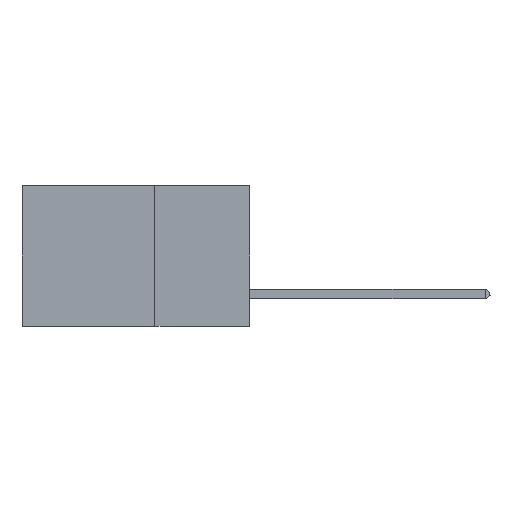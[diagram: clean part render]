
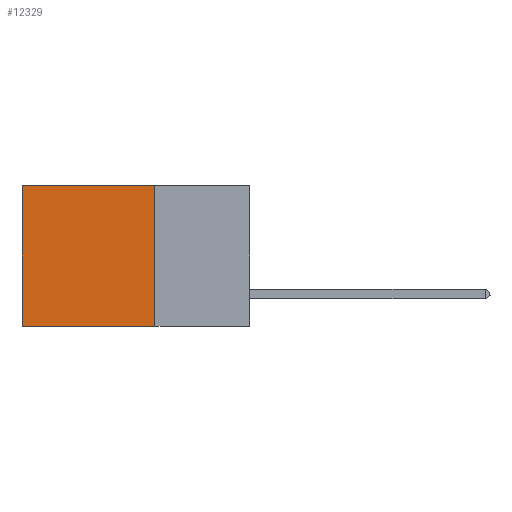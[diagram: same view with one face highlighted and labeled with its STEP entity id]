
A CAD part, left-side view. The second image highlights one B-rep face of the part: STEP entity #12329.
In plain terms, the highlighted planar face has unit normal (-1, 0, 0).
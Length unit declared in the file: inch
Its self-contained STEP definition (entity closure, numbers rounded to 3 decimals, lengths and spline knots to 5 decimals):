
#184 = VECTOR ( 'NONE', #36375, 39.37008 ) ;
#1057 = VERTEX_POINT ( 'NONE', #8124 ) ;
#3148 = AXIS2_PLACEMENT_3D ( 'NONE', #3302, #5001, #36718 ) ;
#3302 = CARTESIAN_POINT ( 'NONE',  ( 0.2875, 0.25, 0. ) ) ;
#3563 = LINE ( 'NONE', #32785, #184 ) ;
#3978 = VERTEX_POINT ( 'NONE', #33314 ) ;
#4868 = DIRECTION ( 'NONE',  ( 0., 0., -1. ) ) ;
#5001 = DIRECTION ( 'NONE',  ( 1., 0., 0. ) ) ;
#5904 = DIRECTION ( 'NONE',  ( 0., 1., 0. ) ) ;
#8124 = CARTESIAN_POINT ( 'NONE',  ( 0.2875, 0.25, -0.37 ) ) ;
#9807 = VERTEX_POINT ( 'NONE', #43853 ) ;
#12329 = ADVANCED_FACE ( 'NONE', ( #24582 ), #19595, .F. ) ;
#13086 = VECTOR ( 'NONE', #5904, 39.37008 ) ;
#13516 = LINE ( 'NONE', #33760, #33788 ) ;
#13643 = VERTEX_POINT ( 'NONE', #44103 ) ;
#16789 = VECTOR ( 'NONE', #41852, 39.37008 ) ;
#19595 = PLANE ( 'NONE',  #3148 ) ;
#22718 = LINE ( 'NONE', #35078, #13086 ) ;
#22846 = EDGE_CURVE ( 'NONE', #3978, #1057, #44266, .T. ) ;
#24582 = FACE_OUTER_BOUND ( 'NONE', #34181, .T. ) ;
#29083 = EDGE_CURVE ( 'NONE', #3978, #9807, #3563, .T. ) ;
#32785 = CARTESIAN_POINT ( 'NONE',  ( 0.2875, 0.25, 0. ) ) ;
#33314 = CARTESIAN_POINT ( 'NONE',  ( 0.2875, 0.25, 0. ) ) ;
#33760 = CARTESIAN_POINT ( 'NONE',  ( 0.2875, 0.6, 0. ) ) ;
#33788 = VECTOR ( 'NONE', #4868, 39.37008 ) ;
#34181 = EDGE_LOOP ( 'NONE', ( #44430, #35342, #35386, #44354 ) ) ;
#35078 = CARTESIAN_POINT ( 'NONE',  ( 0.2875, 0.25, -0.37 ) ) ;
#35342 = ORIENTED_EDGE ( 'NONE', *, *, #42157, .F. ) ;
#35386 = ORIENTED_EDGE ( 'NONE', *, *, #22846, .F. ) ;
#36375 = DIRECTION ( 'NONE',  ( 0., 1., 0. ) ) ;
#36718 = DIRECTION ( 'NONE',  ( 0., 0., -1. ) ) ;
#37499 = EDGE_CURVE ( 'NONE', #9807, #13643, #13516, .T. ) ;
#41852 = DIRECTION ( 'NONE',  ( 0., 0., -1. ) ) ;
#41992 = CARTESIAN_POINT ( 'NONE',  ( 0.2875, 0.25, 0. ) ) ;
#42157 = EDGE_CURVE ( 'NONE', #1057, #13643, #22718, .T. ) ;
#43853 = CARTESIAN_POINT ( 'NONE',  ( 0.2875, 0.6, 0. ) ) ;
#44103 = CARTESIAN_POINT ( 'NONE',  ( 0.2875, 0.6, -0.37 ) ) ;
#44266 = LINE ( 'NONE', #41992, #16789 ) ;
#44354 = ORIENTED_EDGE ( 'NONE', *, *, #29083, .T. ) ;
#44430 = ORIENTED_EDGE ( 'NONE', *, *, #37499, .T. ) ;
